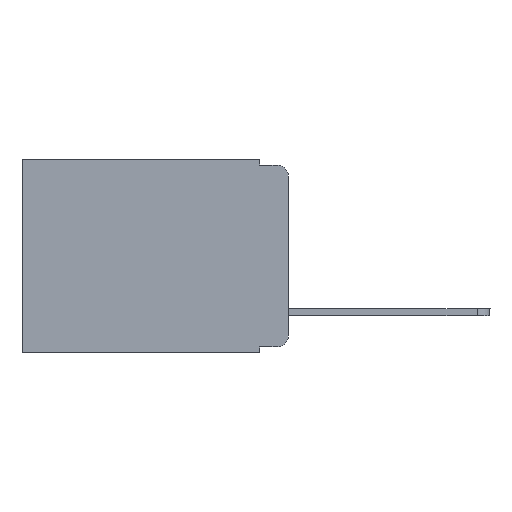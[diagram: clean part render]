
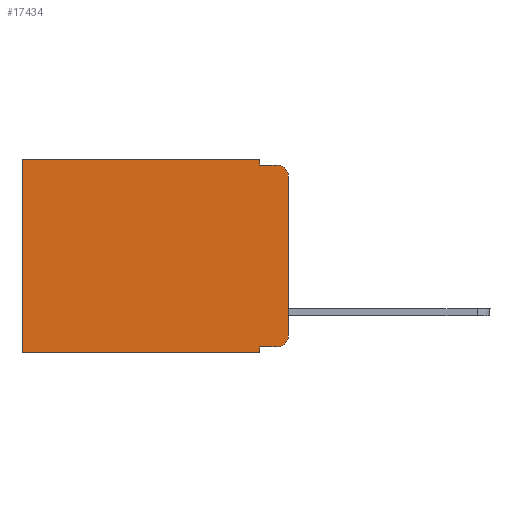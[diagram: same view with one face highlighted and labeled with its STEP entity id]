
A CAD part, left-side view. The second image highlights one B-rep face of the part: STEP entity #17434.
In plain terms, the highlighted planar face has unit normal (-1, 0, 0).
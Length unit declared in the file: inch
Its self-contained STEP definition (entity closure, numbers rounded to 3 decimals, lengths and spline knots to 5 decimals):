
#512 = CARTESIAN_POINT ( 'NONE',  ( 0.298, 0., -0.343 ) ) ;
#598 = CARTESIAN_POINT ( 'NONE',  ( 0.298, 0.473, 0. ) ) ;
#1245 = DIRECTION ( 'NONE',  ( 0., 0., -1. ) ) ;
#1273 = CIRCLE ( 'NONE', #19319, 0.02 ) ;
#1544 = EDGE_LOOP ( 'NONE', ( #4937, #20499, #10505, #4577, #12894, #9145, #9757, #18537, #19605, #16175 ) ) ;
#1897 = VERTEX_POINT ( 'NONE', #17271 ) ;
#2881 = FACE_OUTER_BOUND ( 'NONE', #1544, .T. ) ;
#3376 = CARTESIAN_POINT ( 'NONE',  ( 0.298, 0., -0.313 ) ) ;
#3675 = EDGE_CURVE ( 'NONE', #9837, #13528, #9966, .T. ) ;
#3876 = DIRECTION ( 'NONE',  ( 0., 0., -1. ) ) ;
#4436 = LINE ( 'NONE', #8936, #16253 ) ;
#4571 = CARTESIAN_POINT ( 'NONE',  ( 0.298, 0.051, 0. ) ) ;
#4577 = ORIENTED_EDGE ( 'NONE', *, *, #18403, .F. ) ;
#4693 = CARTESIAN_POINT ( 'NONE',  ( 0.298, 0., 0. ) ) ;
#4937 = ORIENTED_EDGE ( 'NONE', *, *, #9337, .F. ) ;
#5654 = CARTESIAN_POINT ( 'NONE',  ( 0.298, 0., -0.03 ) ) ;
#5757 = VERTEX_POINT ( 'NONE', #18146 ) ;
#5865 = VECTOR ( 'NONE', #1245, 39.37008 ) ;
#5874 = VERTEX_POINT ( 'NONE', #8934 ) ;
#6101 = CARTESIAN_POINT ( 'NONE',  ( 0.298, 0.051, -0.333 ) ) ;
#6245 = VECTOR ( 'NONE', #13522, 39.37008 ) ;
#6360 = LINE ( 'NONE', #4571, #17572 ) ;
#6587 = VECTOR ( 'NONE', #19184, 39.37008 ) ;
#6867 = CARTESIAN_POINT ( 'NONE',  ( 0.298, 0.02, -0.03 ) ) ;
#6936 = VERTEX_POINT ( 'NONE', #3376 ) ;
#7225 = EDGE_CURVE ( 'NONE', #8179, #5874, #17746, .T. ) ;
#8179 = VERTEX_POINT ( 'NONE', #21430 ) ;
#8259 = DIRECTION ( 'NONE',  ( 0., -1., 0. ) ) ;
#8624 = CARTESIAN_POINT ( 'NONE',  ( 0.298, 0.02, -0.01 ) ) ;
#8934 = CARTESIAN_POINT ( 'NONE',  ( 0.298, 0.02, -0.333 ) ) ;
#8936 = CARTESIAN_POINT ( 'NONE',  ( 0.298, 0.051, 0. ) ) ;
#9145 = ORIENTED_EDGE ( 'NONE', *, *, #3675, .T. ) ;
#9337 = EDGE_CURVE ( 'NONE', #15636, #6936, #14793, .T. ) ;
#9472 = EDGE_CURVE ( 'NONE', #1897, #14754, #15538, .T. ) ;
#9757 = ORIENTED_EDGE ( 'NONE', *, *, #12911, .F. ) ;
#9837 = VERTEX_POINT ( 'NONE', #598 ) ;
#9886 = CARTESIAN_POINT ( 'NONE',  ( 0.298, 0.051, -0.01 ) ) ;
#9915 = DIRECTION ( 'NONE',  ( -1., 0., 0. ) ) ;
#9966 = LINE ( 'NONE', #10231, #6245 ) ;
#10231 = CARTESIAN_POINT ( 'NONE',  ( 0.298, 0.473, 0. ) ) ;
#10322 = DIRECTION ( 'NONE',  ( 0., 0., -1. ) ) ;
#10473 = DIRECTION ( 'NONE',  ( 1., 0., 0. ) ) ;
#10505 = ORIENTED_EDGE ( 'NONE', *, *, #9472, .F. ) ;
#10538 = DIRECTION ( 'NONE',  ( 0., 1., 0. ) ) ;
#11038 = LINE ( 'NONE', #512, #6587 ) ;
#11145 = DIRECTION ( 'NONE',  ( 0., 0., -1. ) ) ;
#11272 = AXIS2_PLACEMENT_3D ( 'NONE', #17144, #10473, #20716 ) ;
#11454 = CARTESIAN_POINT ( 'NONE',  ( 0.298, 0.473, -0.343 ) ) ;
#12247 = AXIS2_PLACEMENT_3D ( 'NONE', #6867, #18574, #10322 ) ;
#12580 = EDGE_CURVE ( 'NONE', #8179, #13583, #4436, .T. ) ;
#12894 = ORIENTED_EDGE ( 'NONE', *, *, #15461, .T. ) ;
#12911 = EDGE_CURVE ( 'NONE', #13583, #13528, #11038, .T. ) ;
#12980 = CARTESIAN_POINT ( 'NONE',  ( 0.298, 0.051, -0.343 ) ) ;
#13089 = DIRECTION ( 'NONE',  ( 0., 0., -1. ) ) ;
#13522 = DIRECTION ( 'NONE',  ( 0., 0., -1. ) ) ;
#13528 = VERTEX_POINT ( 'NONE', #11454 ) ;
#13583 = VERTEX_POINT ( 'NONE', #12980 ) ;
#14754 = VERTEX_POINT ( 'NONE', #8624 ) ;
#14793 = LINE ( 'NONE', #4693, #5865 ) ;
#15461 = EDGE_CURVE ( 'NONE', #5757, #9837, #18188, .T. ) ;
#15538 = LINE ( 'NONE', #9886, #20498 ) ;
#15636 = VERTEX_POINT ( 'NONE', #5654 ) ;
#16175 = ORIENTED_EDGE ( 'NONE', *, *, #18441, .T. ) ;
#16253 = VECTOR ( 'NONE', #3876, 39.37008 ) ;
#17144 = CARTESIAN_POINT ( 'NONE',  ( 0.298, 0., 0. ) ) ;
#17271 = CARTESIAN_POINT ( 'NONE',  ( 0.298, 0.051, -0.01 ) ) ;
#17434 = ADVANCED_FACE ( 'NONE', ( #2881 ), #18731, .F. ) ;
#17572 = VECTOR ( 'NONE', #11145, 39.37008 ) ;
#17746 = LINE ( 'NONE', #6101, #18262 ) ;
#17940 = EDGE_CURVE ( 'NONE', #15636, #14754, #20169, .T. ) ;
#18146 = CARTESIAN_POINT ( 'NONE',  ( 0.298, 0.051, 0. ) ) ;
#18188 = LINE ( 'NONE', #20290, #20019 ) ;
#18262 = VECTOR ( 'NONE', #19438, 39.37008 ) ;
#18403 = EDGE_CURVE ( 'NONE', #5757, #1897, #6360, .T. ) ;
#18441 = EDGE_CURVE ( 'NONE', #5874, #6936, #1273, .T. ) ;
#18537 = ORIENTED_EDGE ( 'NONE', *, *, #12580, .F. ) ;
#18574 = DIRECTION ( 'NONE',  ( -1., 0., 0. ) ) ;
#18731 = PLANE ( 'NONE',  #11272 ) ;
#19184 = DIRECTION ( 'NONE',  ( 0., 1., 0. ) ) ;
#19319 = AXIS2_PLACEMENT_3D ( 'NONE', #19858, #9915, #13089 ) ;
#19438 = DIRECTION ( 'NONE',  ( 0., -1., 0. ) ) ;
#19605 = ORIENTED_EDGE ( 'NONE', *, *, #7225, .T. ) ;
#19858 = CARTESIAN_POINT ( 'NONE',  ( 0.298, 0.02, -0.313 ) ) ;
#20019 = VECTOR ( 'NONE', #10538, 39.37008 ) ;
#20169 = CIRCLE ( 'NONE', #12247, 0.02 ) ;
#20290 = CARTESIAN_POINT ( 'NONE',  ( 0.298, 0., 0. ) ) ;
#20498 = VECTOR ( 'NONE', #8259, 39.37008 ) ;
#20499 = ORIENTED_EDGE ( 'NONE', *, *, #17940, .T. ) ;
#20716 = DIRECTION ( 'NONE',  ( 0., 0., -1. ) ) ;
#21430 = CARTESIAN_POINT ( 'NONE',  ( 0.298, 0.051, -0.333 ) ) ;
